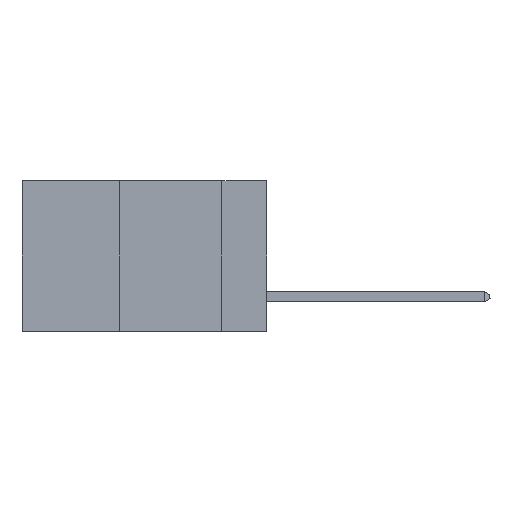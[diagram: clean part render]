
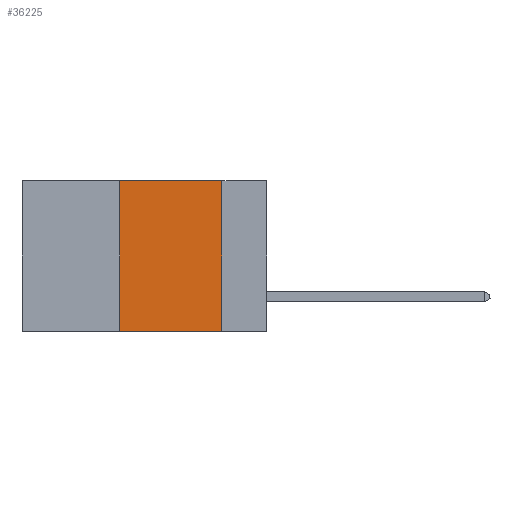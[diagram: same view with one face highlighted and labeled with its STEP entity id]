
A CAD part, left-side view. The second image highlights one B-rep face of the part: STEP entity #36225.
In plain terms, the highlighted planar face has unit normal (-1, 0, 0).
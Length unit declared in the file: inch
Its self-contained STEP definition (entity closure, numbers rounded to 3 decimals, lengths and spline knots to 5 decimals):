
#651 = DIRECTION ( 'NONE',  ( 0., 0., 1. ) ) ;
#972 = VERTEX_POINT ( 'NONE', #33681 ) ;
#1215 = CARTESIAN_POINT ( 'NONE',  ( 0., 0.11, 0. ) ) ;
#3690 = DIRECTION ( 'NONE',  ( 0., 0., -1. ) ) ;
#4318 = ORIENTED_EDGE ( 'NONE', *, *, #15749, .F. ) ;
#4923 = VERTEX_POINT ( 'NONE', #11680 ) ;
#5544 = VERTEX_POINT ( 'NONE', #12942 ) ;
#5726 = PLANE ( 'NONE',  #29025 ) ;
#6586 = CARTESIAN_POINT ( 'NONE',  ( 0., 0.11, -0.37 ) ) ;
#9724 = ORIENTED_EDGE ( 'NONE', *, *, #24438, .T. ) ;
#11680 = CARTESIAN_POINT ( 'NONE',  ( 0., 0.36, 0. ) ) ;
#12010 = VECTOR ( 'NONE', #30577, 39.37008 ) ;
#12318 = DIRECTION ( 'NONE',  ( 0., -1., 0. ) ) ;
#12942 = CARTESIAN_POINT ( 'NONE',  ( 0., 0.36, -0.37 ) ) ;
#14697 = VERTEX_POINT ( 'NONE', #6586 ) ;
#15749 = EDGE_CURVE ( 'NONE', #5544, #4923, #23729, .T. ) ;
#16214 = EDGE_CURVE ( 'NONE', #972, #14697, #28683, .T. ) ;
#17711 = DIRECTION ( 'NONE',  ( 1., 0., 0. ) ) ;
#17757 = EDGE_LOOP ( 'NONE', ( #36336, #34073, #4318, #9724 ) ) ;
#23729 = LINE ( 'NONE', #34539, #24194 ) ;
#23885 = CARTESIAN_POINT ( 'NONE',  ( 0., 0.6, -0.37 ) ) ;
#24194 = VECTOR ( 'NONE', #651, 39.37008 ) ;
#24438 = EDGE_CURVE ( 'NONE', #5544, #14697, #29948, .T. ) ;
#25586 = LINE ( 'NONE', #33746, #12010 ) ;
#26527 = CARTESIAN_POINT ( 'NONE',  ( 0., 0.6, 0. ) ) ;
#27777 = VECTOR ( 'NONE', #30490, 39.37008 ) ;
#28683 = LINE ( 'NONE', #1215, #27777 ) ;
#29025 = AXIS2_PLACEMENT_3D ( 'NONE', #26527, #17711, #3690 ) ;
#29851 = EDGE_CURVE ( 'NONE', #4923, #972, #25586, .T. ) ;
#29948 = LINE ( 'NONE', #23885, #32640 ) ;
#30490 = DIRECTION ( 'NONE',  ( 0., 0., -1. ) ) ;
#30577 = DIRECTION ( 'NONE',  ( 0., -1., 0. ) ) ;
#32640 = VECTOR ( 'NONE', #12318, 39.37008 ) ;
#33681 = CARTESIAN_POINT ( 'NONE',  ( 0., 0.11, 0. ) ) ;
#33746 = CARTESIAN_POINT ( 'NONE',  ( 0., 0.6, 0. ) ) ;
#34073 = ORIENTED_EDGE ( 'NONE', *, *, #29851, .F. ) ;
#34539 = CARTESIAN_POINT ( 'NONE',  ( 0., 0.36, 0. ) ) ;
#36084 = FACE_OUTER_BOUND ( 'NONE', #17757, .T. ) ;
#36225 = ADVANCED_FACE ( 'NONE', ( #36084 ), #5726, .F. ) ;
#36336 = ORIENTED_EDGE ( 'NONE', *, *, #16214, .F. ) ;
